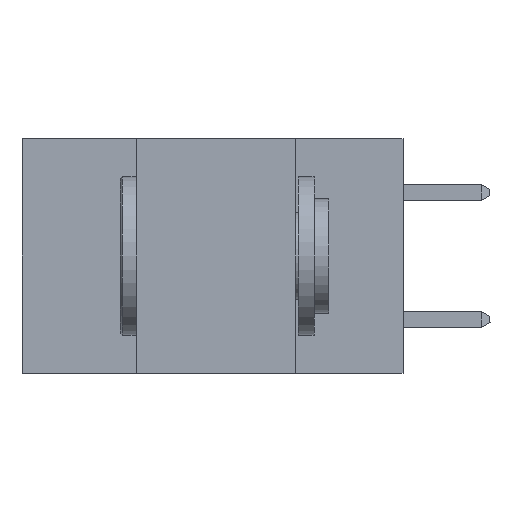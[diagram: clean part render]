
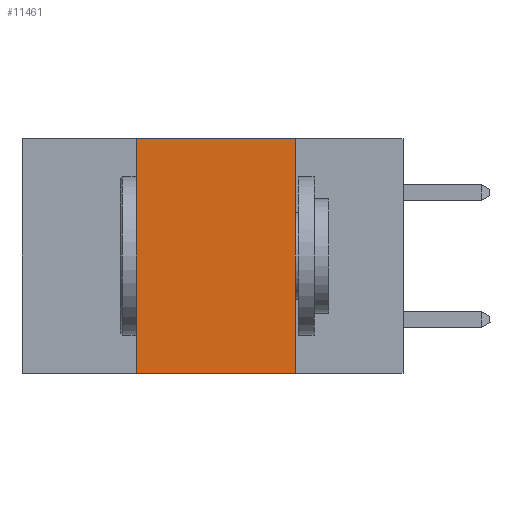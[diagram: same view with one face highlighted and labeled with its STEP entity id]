
A CAD part, left-side view. The second image highlights one B-rep face of the part: STEP entity #11461.
In plain terms, the highlighted planar face has unit normal (-1, 0, 0).
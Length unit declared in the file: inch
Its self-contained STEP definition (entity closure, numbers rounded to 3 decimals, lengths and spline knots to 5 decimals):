
#614 = ORIENTED_EDGE ( 'NONE', *, *, #31026, .F. ) ;
#1205 = CARTESIAN_POINT ( 'NONE',  ( 0., 0.42, -0.37 ) ) ;
#2113 = DIRECTION ( 'NONE',  ( 0., 0., -1. ) ) ;
#2397 = EDGE_CURVE ( 'NONE', #6220, #7966, #39698, .T. ) ;
#2650 = CARTESIAN_POINT ( 'NONE',  ( 0., 0.42, 0. ) ) ;
#4981 = EDGE_CURVE ( 'NONE', #6220, #7262, #32690, .T. ) ;
#6214 = EDGE_LOOP ( 'NONE', ( #36849, #614, #9950, #8567 ) ) ;
#6220 = VERTEX_POINT ( 'NONE', #1205 ) ;
#7262 = VERTEX_POINT ( 'NONE', #2650 ) ;
#7966 = VERTEX_POINT ( 'NONE', #38517 ) ;
#8567 = ORIENTED_EDGE ( 'NONE', *, *, #2397, .T. ) ;
#9950 = ORIENTED_EDGE ( 'NONE', *, *, #4981, .F. ) ;
#10699 = CARTESIAN_POINT ( 'NONE',  ( 0., 0.17, 0. ) ) ;
#11461 = ADVANCED_FACE ( 'NONE', ( #25278 ), #17241, .F. ) ;
#13053 = LINE ( 'NONE', #10699, #30042 ) ;
#17241 = PLANE ( 'NONE',  #30396 ) ;
#18124 = CARTESIAN_POINT ( 'NONE',  ( 0., 0.42, 0. ) ) ;
#18394 = DIRECTION ( 'NONE',  ( 0., 0., 1. ) ) ;
#18787 = CARTESIAN_POINT ( 'NONE',  ( 0., 0.17, 0. ) ) ;
#19123 = VECTOR ( 'NONE', #19177, 39.37008 ) ;
#19177 = DIRECTION ( 'NONE',  ( 0., -1., 0. ) ) ;
#19899 = DIRECTION ( 'NONE',  ( 0., 0., -1. ) ) ;
#20733 = DIRECTION ( 'NONE',  ( 1., 0., 0. ) ) ;
#25238 = VERTEX_POINT ( 'NONE', #18787 ) ;
#25278 = FACE_OUTER_BOUND ( 'NONE', #6214, .T. ) ;
#27431 = LINE ( 'NONE', #28414, #19123 ) ;
#27588 = VECTOR ( 'NONE', #39673, 39.37008 ) ;
#28414 = CARTESIAN_POINT ( 'NONE',  ( 0., 0.6, 0. ) ) ;
#30042 = VECTOR ( 'NONE', #19899, 39.37008 ) ;
#30396 = AXIS2_PLACEMENT_3D ( 'NONE', #33026, #20733, #2113 ) ;
#31026 = EDGE_CURVE ( 'NONE', #7262, #25238, #27431, .T. ) ;
#32690 = LINE ( 'NONE', #18124, #33669 ) ;
#33026 = CARTESIAN_POINT ( 'NONE',  ( 0., 0.6, 0. ) ) ;
#33478 = CARTESIAN_POINT ( 'NONE',  ( 0., 0.6, -0.37 ) ) ;
#33669 = VECTOR ( 'NONE', #18394, 39.37008 ) ;
#34962 = EDGE_CURVE ( 'NONE', #25238, #7966, #13053, .T. ) ;
#36849 = ORIENTED_EDGE ( 'NONE', *, *, #34962, .F. ) ;
#38517 = CARTESIAN_POINT ( 'NONE',  ( 0., 0.17, -0.37 ) ) ;
#39673 = DIRECTION ( 'NONE',  ( 0., -1., 0. ) ) ;
#39698 = LINE ( 'NONE', #33478, #27588 ) ;
